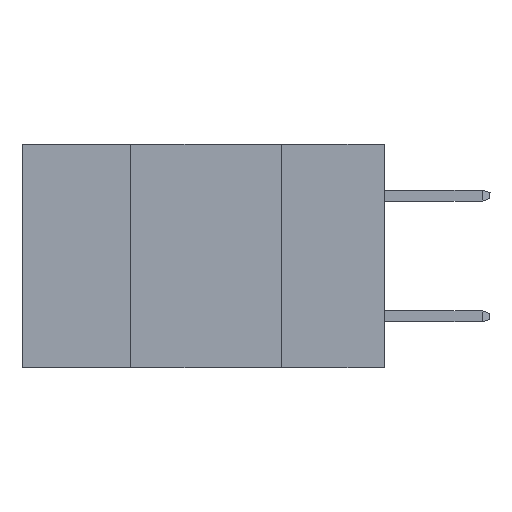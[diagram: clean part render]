
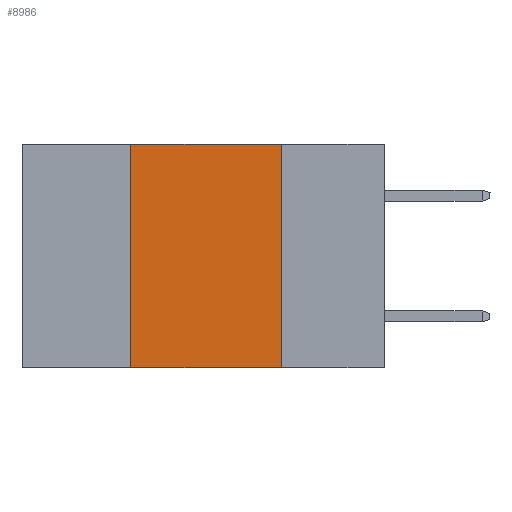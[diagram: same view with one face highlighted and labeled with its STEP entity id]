
A CAD part, left-side view. The second image highlights one B-rep face of the part: STEP entity #8986.
In plain terms, the highlighted planar face has unit normal (-1, 0, 0).
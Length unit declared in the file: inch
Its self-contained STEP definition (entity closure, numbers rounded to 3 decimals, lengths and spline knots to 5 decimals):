
#789 = VECTOR ( 'NONE', #30696, 39.37008 ) ;
#1969 = CARTESIAN_POINT ( 'NONE',  ( 0., 0.42, 0. ) ) ;
#2094 = CARTESIAN_POINT ( 'NONE',  ( 0., 0.6, 0. ) ) ;
#2635 = VECTOR ( 'NONE', #32960, 39.37008 ) ;
#3713 = EDGE_CURVE ( 'NONE', #11403, #14977, #27916, .T. ) ;
#4546 = FACE_OUTER_BOUND ( 'NONE', #30855, .T. ) ;
#4745 = DIRECTION ( 'NONE',  ( 1., 0., 0. ) ) ;
#8986 = ADVANCED_FACE ( 'NONE', ( #4546 ), #17633, .F. ) ;
#9596 = LINE ( 'NONE', #20199, #2635 ) ;
#11403 = VERTEX_POINT ( 'NONE', #26365 ) ;
#12443 = EDGE_CURVE ( 'NONE', #15419, #14977, #9596, .T. ) ;
#14699 = VECTOR ( 'NONE', #17511, 39.37008 ) ;
#14977 = VERTEX_POINT ( 'NONE', #29604 ) ;
#15267 = CARTESIAN_POINT ( 'NONE',  ( 0., 0.6, 0. ) ) ;
#15419 = VERTEX_POINT ( 'NONE', #28611 ) ;
#15449 = CARTESIAN_POINT ( 'NONE',  ( 0., 0.17, 0. ) ) ;
#15897 = EDGE_CURVE ( 'NONE', #15419, #24553, #20770, .T. ) ;
#16723 = EDGE_CURVE ( 'NONE', #24553, #11403, #28377, .T. ) ;
#17511 = DIRECTION ( 'NONE',  ( 0., 0., 1. ) ) ;
#17633 = PLANE ( 'NONE',  #31076 ) ;
#17806 = ORIENTED_EDGE ( 'NONE', *, *, #12443, .T. ) ;
#20199 = CARTESIAN_POINT ( 'NONE',  ( 0., 0.6, -0.37 ) ) ;
#20770 = LINE ( 'NONE', #1969, #14699 ) ;
#21058 = ORIENTED_EDGE ( 'NONE', *, *, #3713, .F. ) ;
#22513 = ORIENTED_EDGE ( 'NONE', *, *, #16723, .F. ) ;
#22852 = DIRECTION ( 'NONE',  ( 0., 0., -1. ) ) ;
#23214 = CARTESIAN_POINT ( 'NONE',  ( 0., 0.42, 0. ) ) ;
#24553 = VERTEX_POINT ( 'NONE', #23214 ) ;
#26365 = CARTESIAN_POINT ( 'NONE',  ( 0., 0.17, 0. ) ) ;
#27636 = DIRECTION ( 'NONE',  ( 0., 0., -1. ) ) ;
#27916 = LINE ( 'NONE', #15449, #28718 ) ;
#28377 = LINE ( 'NONE', #15267, #789 ) ;
#28611 = CARTESIAN_POINT ( 'NONE',  ( 0., 0.42, -0.37 ) ) ;
#28718 = VECTOR ( 'NONE', #27636, 39.37008 ) ;
#29604 = CARTESIAN_POINT ( 'NONE',  ( 0., 0.17, -0.37 ) ) ;
#30696 = DIRECTION ( 'NONE',  ( 0., -1., 0. ) ) ;
#30855 = EDGE_LOOP ( 'NONE', ( #21058, #22513, #33342, #17806 ) ) ;
#31076 = AXIS2_PLACEMENT_3D ( 'NONE', #2094, #4745, #22852 ) ;
#32960 = DIRECTION ( 'NONE',  ( 0., -1., 0. ) ) ;
#33342 = ORIENTED_EDGE ( 'NONE', *, *, #15897, .F. ) ;
